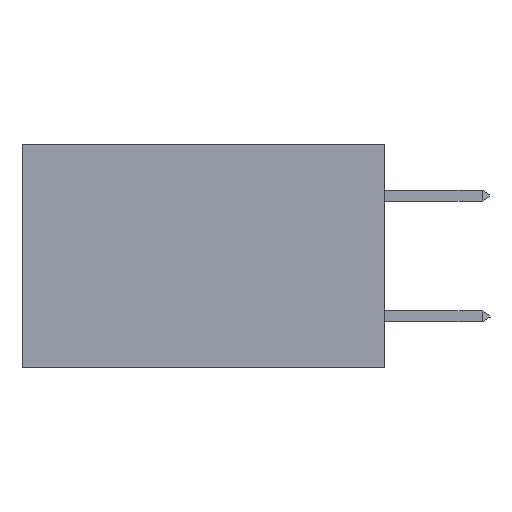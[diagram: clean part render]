
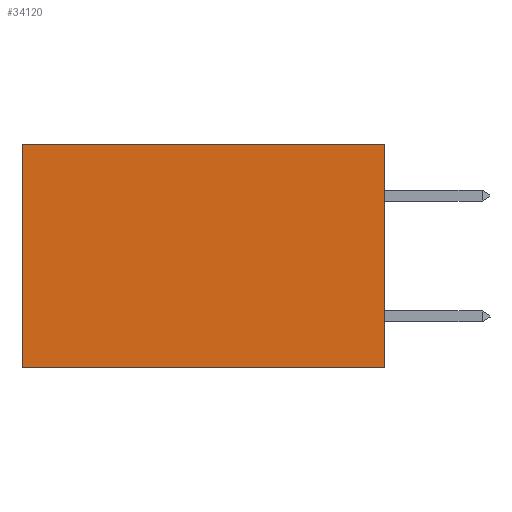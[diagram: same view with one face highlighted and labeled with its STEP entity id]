
A CAD part, left-side view. The second image highlights one B-rep face of the part: STEP entity #34120.
In plain terms, the highlighted planar face has unit normal (-1, 0, 0).
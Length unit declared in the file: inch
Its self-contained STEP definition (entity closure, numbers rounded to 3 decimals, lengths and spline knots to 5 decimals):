
#386 = LINE ( 'NONE', #946, #25221 ) ;
#603 = VERTEX_POINT ( 'NONE', #21560 ) ;
#946 = CARTESIAN_POINT ( 'NONE',  ( 0.2875, 0.6, 0. ) ) ;
#5672 = LINE ( 'NONE', #18360, #27997 ) ;
#5905 = DIRECTION ( 'NONE',  ( 1., 0., 0. ) ) ;
#6026 = EDGE_LOOP ( 'NONE', ( #24077, #9997, #21103, #16281 ) ) ;
#6184 = DIRECTION ( 'NONE',  ( 0., 0., -1. ) ) ;
#9771 = LINE ( 'NONE', #13480, #40667 ) ;
#9997 = ORIENTED_EDGE ( 'NONE', *, *, #36219, .F. ) ;
#12543 = FACE_OUTER_BOUND ( 'NONE', #6026, .T. ) ;
#12705 = CARTESIAN_POINT ( 'NONE',  ( 0.2875, 0., 0. ) ) ;
#13480 = CARTESIAN_POINT ( 'NONE',  ( 0.2875, 0., -0.37 ) ) ;
#16281 = ORIENTED_EDGE ( 'NONE', *, *, #25799, .T. ) ;
#18360 = CARTESIAN_POINT ( 'NONE',  ( 0.2875, 0., 0. ) ) ;
#20141 = DIRECTION ( 'NONE',  ( 0., 1., 0. ) ) ;
#21103 = ORIENTED_EDGE ( 'NONE', *, *, #25661, .F. ) ;
#21560 = CARTESIAN_POINT ( 'NONE',  ( 0.2875, 0.6, 0. ) ) ;
#22011 = VERTEX_POINT ( 'NONE', #38617 ) ;
#22024 = VERTEX_POINT ( 'NONE', #22502 ) ;
#22502 = CARTESIAN_POINT ( 'NONE',  ( 0.2875, 0., 0. ) ) ;
#22605 = PLANE ( 'NONE',  #35001 ) ;
#22731 = DIRECTION ( 'NONE',  ( 0., 1., 0. ) ) ;
#23630 = DIRECTION ( 'NONE',  ( 0., 0., -1. ) ) ;
#24077 = ORIENTED_EDGE ( 'NONE', *, *, #33513, .T. ) ;
#25221 = VECTOR ( 'NONE', #23630, 39.37008 ) ;
#25661 = EDGE_CURVE ( 'NONE', #22024, #35703, #5672, .T. ) ;
#25799 = EDGE_CURVE ( 'NONE', #22024, #603, #36041, .T. ) ;
#27997 = VECTOR ( 'NONE', #37872, 39.37008 ) ;
#28930 = VECTOR ( 'NONE', #22731, 39.37008 ) ;
#29345 = CARTESIAN_POINT ( 'NONE',  ( 0.2875, 0., 0. ) ) ;
#33513 = EDGE_CURVE ( 'NONE', #603, #22011, #386, .T. ) ;
#34120 = ADVANCED_FACE ( 'NONE', ( #12543 ), #22605, .F. ) ;
#35001 = AXIS2_PLACEMENT_3D ( 'NONE', #12705, #5905, #6184 ) ;
#35703 = VERTEX_POINT ( 'NONE', #40264 ) ;
#36041 = LINE ( 'NONE', #29345, #28930 ) ;
#36219 = EDGE_CURVE ( 'NONE', #35703, #22011, #9771, .T. ) ;
#37872 = DIRECTION ( 'NONE',  ( 0., 0., -1. ) ) ;
#38617 = CARTESIAN_POINT ( 'NONE',  ( 0.2875, 0.6, -0.37 ) ) ;
#40264 = CARTESIAN_POINT ( 'NONE',  ( 0.2875, 0., -0.37 ) ) ;
#40667 = VECTOR ( 'NONE', #20141, 39.37008 ) ;
